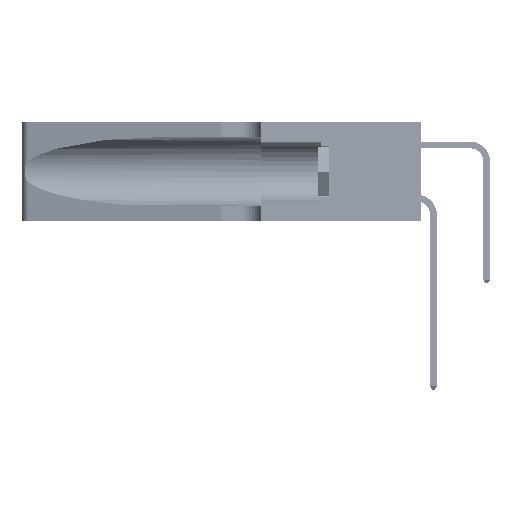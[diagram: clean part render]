
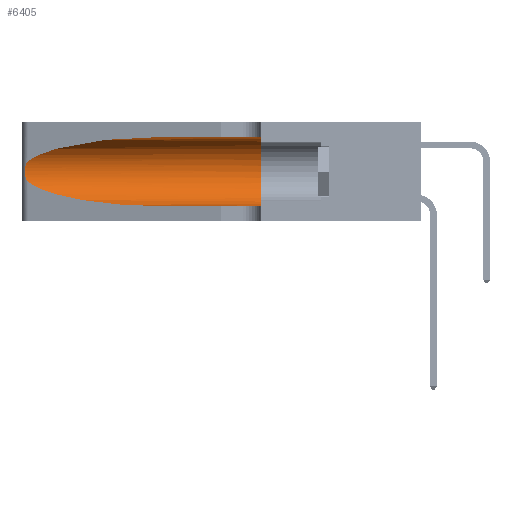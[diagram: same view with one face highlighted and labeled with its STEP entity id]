
A CAD part, left-side view. The second image highlights one B-rep face of the part: STEP entity #6405.
In plain terms, the highlighted cylindrical face has radius 3.308 mm (diameter 6.617 mm), a partial arc.
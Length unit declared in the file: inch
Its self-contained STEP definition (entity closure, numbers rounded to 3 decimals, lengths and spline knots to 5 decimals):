
#297 = FACE_OUTER_BOUND ( 'NONE', #28679, .T. ) ;
#455 = LINE ( 'NONE', #51714, #7504 ) ;
#1235 = VECTOR ( 'NONE', #15864, 39.37008 ) ;
#2051 = CARTESIAN_POINT ( 'NONE',  ( 0.2373, 1.15595, 0.08982 ) ) ;
#2200 = CARTESIAN_POINT ( 'NONE',  ( 0.26075, 1.23896, 0.178 ) ) ;
#3275 = ORIENTED_EDGE ( 'NONE', *, *, #11492, .F. ) ;
#4851 =( BOUNDED_CURVE ( )  B_SPLINE_CURVE ( 3, ( #51097, #2051, #30716, #43039 ),
 .UNSPECIFIED., .F., .F. ) 
 B_SPLINE_CURVE_WITH_KNOTS ( ( 4, 4 ),
 ( 3.44316, 4.71239 ),
 .UNSPECIFIED. ) 
 CURVE ( )  GEOMETRIC_REPRESENTATION_ITEM ( )  RATIONAL_B_SPLINE_CURVE ( ( 1., 0.87, 0.87, 1. ) ) 
 REPRESENTATION_ITEM ( '' )  );
#5150 = CARTESIAN_POINT ( 'NONE',  ( 0.25487, 1.22718, 0.14631 ) ) ;
#6192 = CARTESIAN_POINT ( 'NONE',  ( 0.1305, 0.72297, 0.31525 ) ) ;
#6405 = ADVANCED_FACE ( 'NONE', ( #297 ), #42578, .F. ) ;
#6648 = EDGE_CURVE ( 'NONE', #48108, #34149, #18224, .T. ) ;
#6660 = CARTESIAN_POINT ( 'NONE',  ( 0.25487, 1.22718, 0.22369 ) ) ;
#7504 = VECTOR ( 'NONE', #51873, 39.37008 ) ;
#10325 = ORIENTED_EDGE ( 'NONE', *, *, #41746, .T. ) ;
#10751 = CARTESIAN_POINT ( 'NONE',  ( 0.25789, 1.23486, 0.15765 ) ) ;
#11438 = LINE ( 'NONE', #15514, #1235 ) ;
#11492 = EDGE_CURVE ( 'NONE', #19759, #48108, #11438, .T. ) ;
#12496 = CARTESIAN_POINT ( 'NONE',  ( 0.18966, 0.96281, 0.31525 ) ) ;
#15514 = CARTESIAN_POINT ( 'NONE',  ( 0.1305, 1.61858, 0.31525 ) ) ;
#15864 = DIRECTION ( 'NONE',  ( 0., -1., 0. ) ) ;
#16633 = CARTESIAN_POINT ( 'NONE',  ( 0.25487, 1.22718, 0.22369 ) ) ;
#16814 = CARTESIAN_POINT ( 'NONE',  ( 0.2373, 1.15595, 0.28018 ) ) ;
#18067 = CARTESIAN_POINT ( 'NONE',  ( 0.1305, 0.35, 0.05475 ) ) ;
#18224 = CIRCLE ( 'NONE', #42870, 0.13025 ) ;
#18514 = CARTESIAN_POINT ( 'NONE',  ( 0.25854, 1.2359, 0.20912 ) ) ;
#18869 = VERTEX_POINT ( 'NONE', #34383 ) ;
#18947 = VERTEX_POINT ( 'NONE', #25986 ) ;
#19759 = VERTEX_POINT ( 'NONE', #6192 ) ;
#22013 = EDGE_CURVE ( 'NONE', #19759, #18869, #37353, .T. ) ;
#22180 = VERTEX_POINT ( 'NONE', #5150 ) ;
#22632 = CARTESIAN_POINT ( 'NONE',  ( 0.26075, 1.23896, 0.19203 ) ) ;
#23153 = DIRECTION ( 'NONE',  ( 0., 0., 1. ) ) ;
#25986 = CARTESIAN_POINT ( 'NONE',  ( 0.1305, 0.72297, 0.05475 ) ) ;
#27026 = ORIENTED_EDGE ( 'NONE', *, *, #22013, .T. ) ;
#27119 = CARTESIAN_POINT ( 'NONE',  ( 0.1305, 0.35, 0.185 ) ) ;
#27446 = CARTESIAN_POINT ( 'NONE',  ( 0.25639, 1.23184, 0.21858 ) ) ;
#28060 = CARTESIAN_POINT ( 'NONE',  ( 0.1305, 0.35, 0.31525 ) ) ;
#28679 = EDGE_LOOP ( 'NONE', ( #27026, #10325, #35144, #30819, #32429, #3275 ) ) ;
#30716 = CARTESIAN_POINT ( 'NONE',  ( 0.18966, 0.96281, 0.05475 ) ) ;
#30819 = ORIENTED_EDGE ( 'NONE', *, *, #48737, .T. ) ;
#30860 = CARTESIAN_POINT ( 'NONE',  ( 0.25856, 1.23593, 0.16098 ) ) ;
#32429 = ORIENTED_EDGE ( 'NONE', *, *, #6648, .F. ) ;
#33417 = DIRECTION ( 'NONE',  ( 0., 0., -1. ) ) ;
#33771 = CARTESIAN_POINT ( 'NONE',  ( 0.1305, 1.61858, 0.185 ) ) ;
#34149 = VERTEX_POINT ( 'NONE', #18067 ) ;
#34383 = CARTESIAN_POINT ( 'NONE',  ( 0.25487, 1.22718, 0.22369 ) ) ;
#34975 = CARTESIAN_POINT ( 'NONE',  ( 0.25639, 1.23186, 0.15144 ) ) ;
#35144 = ORIENTED_EDGE ( 'NONE', *, *, #36689, .T. ) ;
#35148 = CARTESIAN_POINT ( 'NONE',  ( 0.25787, 1.23484, 0.2124 ) ) ;
#35660 = CARTESIAN_POINT ( 'NONE',  ( 0.26018, 1.23835, 0.19895 ) ) ;
#36689 = EDGE_CURVE ( 'NONE', #22180, #18947, #4851, .T. ) ;
#37353 =( BOUNDED_CURVE ( )  B_SPLINE_CURVE ( 3, ( #41314, #12496, #16814, #16633 ),
 .UNSPECIFIED., .F., .F. ) 
 B_SPLINE_CURVE_WITH_KNOTS ( ( 4, 4 ),
 ( 1.5708, 2.84003 ),
 .UNSPECIFIED. ) 
 CURVE ( )  GEOMETRIC_REPRESENTATION_ITEM ( )  RATIONAL_B_SPLINE_CURVE ( ( 1., 0.87, 0.87, 1. ) ) 
 REPRESENTATION_ITEM ( '' )  );
#38388 = AXIS2_PLACEMENT_3D ( 'NONE', #33771, #41790, #33417 ) ;
#39041 = CARTESIAN_POINT ( 'NONE',  ( 0.25555, 1.22993, 0.14849 ) ) ;
#39630 = B_SPLINE_CURVE_WITH_KNOTS ( 'NONE', 3,
 ( #6660, #51929, #27446, #35148, #18514, #35660, #22632, #2200, #43367, #30860, #10751, #34975, #39041, #43185 ),
 .UNSPECIFIED., .F., .F.,
 ( 4, 2, 2, 2, 2, 2, 4 ),
 ( 0., 0.00027, 0.00053, 0.00107, 0.0016, 0.00187, 0.00214 ),
 .UNSPECIFIED. ) ;
#41314 = CARTESIAN_POINT ( 'NONE',  ( 0.1305, 0.72297, 0.31525 ) ) ;
#41746 = EDGE_CURVE ( 'NONE', #18869, #22180, #39630, .T. ) ;
#41790 = DIRECTION ( 'NONE',  ( 0., -1., 0. ) ) ;
#42578 = CYLINDRICAL_SURFACE ( 'NONE', #38388, 0.13025 ) ;
#42870 = AXIS2_PLACEMENT_3D ( 'NONE', #27119, #43390, #23153 ) ;
#43039 = CARTESIAN_POINT ( 'NONE',  ( 0.1305, 0.72297, 0.05475 ) ) ;
#43185 = CARTESIAN_POINT ( 'NONE',  ( 0.25487, 1.22718, 0.14631 ) ) ;
#43367 = CARTESIAN_POINT ( 'NONE',  ( 0.26017, 1.23833, 0.17102 ) ) ;
#43390 = DIRECTION ( 'NONE',  ( 0., 1., 0. ) ) ;
#48108 = VERTEX_POINT ( 'NONE', #28060 ) ;
#48737 = EDGE_CURVE ( 'NONE', #18947, #34149, #455, .T. ) ;
#51097 = CARTESIAN_POINT ( 'NONE',  ( 0.25487, 1.22718, 0.14631 ) ) ;
#51714 = CARTESIAN_POINT ( 'NONE',  ( 0.1305, 1.61858, 0.05475 ) ) ;
#51873 = DIRECTION ( 'NONE',  ( 0., -1., 0. ) ) ;
#51929 = CARTESIAN_POINT ( 'NONE',  ( 0.25555, 1.22994, 0.2215 ) ) ;
